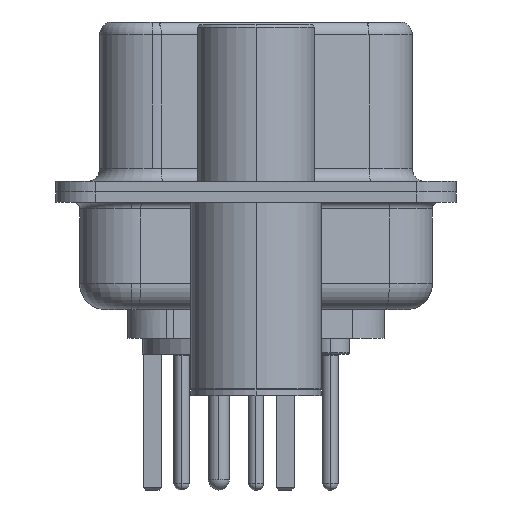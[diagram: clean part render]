
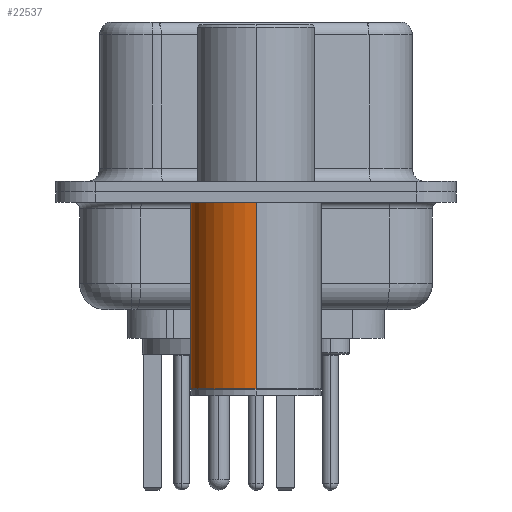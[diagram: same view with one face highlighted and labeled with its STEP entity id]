
A CAD part, left-side view. The second image highlights one B-rep face of the part: STEP entity #22537.
In plain terms, the highlighted cylindrical face has radius 2.5 mm (diameter 5 mm), a partial arc.
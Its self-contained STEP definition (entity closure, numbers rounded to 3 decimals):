
#490 = FACE_OUTER_BOUND ( 'NONE', #6771, .T. ) ;
#3085 = DIRECTION ( 'NONE',  ( 0., 0., 1. ) ) ;
#3247 = CARTESIAN_POINT ( 'NONE',  ( 2.5, 0., 0.581 ) ) ;
#4146 = ORIENTED_EDGE ( 'NONE', *, *, #17300, .T. ) ;
#4888 = CARTESIAN_POINT ( 'NONE',  ( 2.5, 0., -0.4 ) ) ;
#5962 = VECTOR ( 'NONE', #19843, 1000. ) ;
#6025 = CIRCLE ( 'NONE', #28654, 2.5 ) ;
#6771 = EDGE_LOOP ( 'NONE', ( #4146, #17779, #22661, #9249 ) ) ;
#6787 = DIRECTION ( 'NONE',  ( 0., 0., 1. ) ) ;
#7155 = VERTEX_POINT ( 'NONE', #8080 ) ;
#7707 = AXIS2_PLACEMENT_3D ( 'NONE', #28109, #6787, #13857 ) ;
#7802 = CARTESIAN_POINT ( 'NONE',  ( -2.5, 0., -0.4 ) ) ;
#8080 = CARTESIAN_POINT ( 'NONE',  ( 2.5, 0., -7.525 ) ) ;
#8451 = VERTEX_POINT ( 'NONE', #4888 ) ;
#9249 = ORIENTED_EDGE ( 'NONE', *, *, #18405, .F. ) ;
#9254 = VERTEX_POINT ( 'NONE', #7802 ) ;
#9966 = LINE ( 'NONE', #14610, #21865 ) ;
#11166 = DIRECTION ( 'NONE',  ( 0., 0., 1. ) ) ;
#11627 = CYLINDRICAL_SURFACE ( 'NONE', #7707, 2.5 ) ;
#13857 = DIRECTION ( 'NONE',  ( 1., 0., 0. ) ) ;
#14610 = CARTESIAN_POINT ( 'NONE',  ( -2.5, 0., 0.581 ) ) ;
#15704 = CIRCLE ( 'NONE', #21227, 2.5 ) ;
#16985 = DIRECTION ( 'NONE',  ( 0., 0., 1. ) ) ;
#17241 = CARTESIAN_POINT ( 'NONE',  ( 0., 0., -0.4 ) ) ;
#17300 = EDGE_CURVE ( 'NONE', #7155, #29770, #6025, .T. ) ;
#17768 = CARTESIAN_POINT ( 'NONE',  ( -2.5, 0., -7.525 ) ) ;
#17779 = ORIENTED_EDGE ( 'NONE', *, *, #19010, .T. ) ;
#18405 = EDGE_CURVE ( 'NONE', #7155, #8451, #18506, .T. ) ;
#18506 = LINE ( 'NONE', #3247, #5962 ) ;
#19010 = EDGE_CURVE ( 'NONE', #29770, #9254, #9966, .T. ) ;
#19686 = DIRECTION ( 'NONE',  ( 1., 0., 0. ) ) ;
#19843 = DIRECTION ( 'NONE',  ( 0., 0., 1. ) ) ;
#21227 = AXIS2_PLACEMENT_3D ( 'NONE', #17241, #3085, #19686 ) ;
#21634 = EDGE_CURVE ( 'NONE', #8451, #9254, #15704, .T. ) ;
#21865 = VECTOR ( 'NONE', #16985, 1000. ) ;
#22537 = ADVANCED_FACE ( 'NONE', ( #490 ), #11627, .T. ) ;
#22661 = ORIENTED_EDGE ( 'NONE', *, *, #21634, .F. ) ;
#25353 = CARTESIAN_POINT ( 'NONE',  ( 0., 0., -7.525 ) ) ;
#27754 = DIRECTION ( 'NONE',  ( 1., 0., 0. ) ) ;
#28109 = CARTESIAN_POINT ( 'NONE',  ( 0., 0., 0.581 ) ) ;
#28654 = AXIS2_PLACEMENT_3D ( 'NONE', #25353, #11166, #27754 ) ;
#29770 = VERTEX_POINT ( 'NONE', #17768 ) ;
